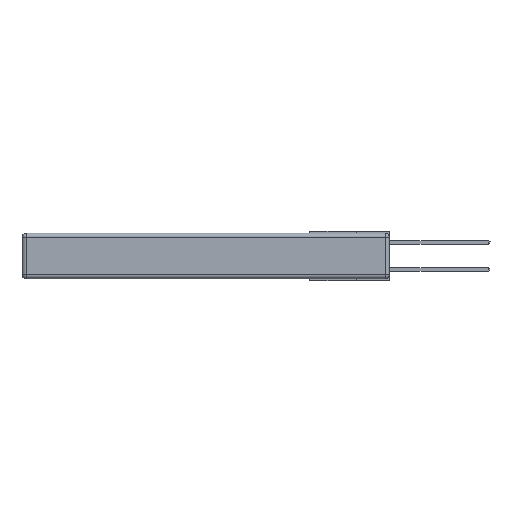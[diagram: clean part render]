
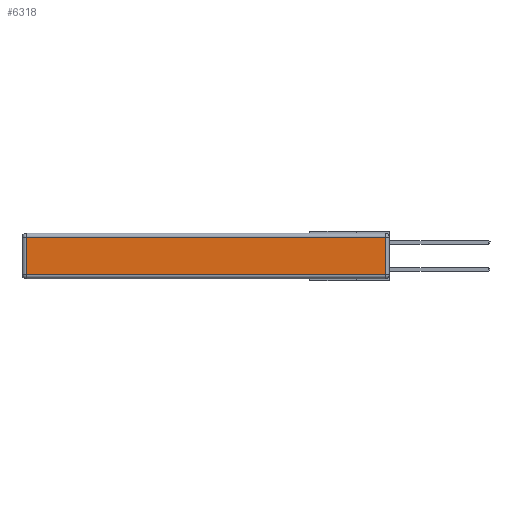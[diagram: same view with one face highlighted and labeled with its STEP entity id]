
A CAD part, left-side view. The second image highlights one B-rep face of the part: STEP entity #6318.
In plain terms, the highlighted planar face has unit normal (-1, 0, 0).
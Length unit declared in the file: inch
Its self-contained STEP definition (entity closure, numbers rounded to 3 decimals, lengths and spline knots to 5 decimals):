
#232 = DIRECTION ( 'NONE',  ( -1., 0., 0. ) ) ;
#442 = AXIS2_PLACEMENT_3D ( 'NONE', #15567, #232, #3858 ) ;
#449 = VECTOR ( 'NONE', #12687, 39.37008 ) ;
#954 = DIRECTION ( 'NONE',  ( 0., 0., -1. ) ) ;
#2299 = VERTEX_POINT ( 'NONE', #6662 ) ;
#2398 = CARTESIAN_POINT ( 'NONE',  ( 0., 0., -0.313 ) ) ;
#2404 = CARTESIAN_POINT ( 'NONE',  ( 0., 2.72, -0.343 ) ) ;
#2431 = EDGE_CURVE ( 'NONE', #2299, #5379, #15868, .T. ) ;
#3386 = FACE_OUTER_BOUND ( 'NONE', #5358, .T. ) ;
#3858 = DIRECTION ( 'NONE',  ( 0., 0., 1. ) ) ;
#4291 = DIRECTION ( 'NONE',  ( 0., 1., 0. ) ) ;
#4744 = EDGE_CURVE ( 'NONE', #13904, #5385, #16327, .T. ) ;
#4854 = EDGE_CURVE ( 'NONE', #5385, #2299, #6262, .T. ) ;
#5204 = PLANE ( 'NONE',  #442 ) ;
#5358 = EDGE_LOOP ( 'NONE', ( #5891, #11018, #9616, #16055 ) ) ;
#5379 = VERTEX_POINT ( 'NONE', #16578 ) ;
#5385 = VERTEX_POINT ( 'NONE', #16473 ) ;
#5401 = DIRECTION ( 'NONE',  ( 0., 0., 1. ) ) ;
#5891 = ORIENTED_EDGE ( 'NONE', *, *, #4744, .T. ) ;
#6262 = LINE ( 'NONE', #11719, #15922 ) ;
#6318 = ADVANCED_FACE ( 'NONE', ( #3386 ), #5204, .T. ) ;
#6662 = CARTESIAN_POINT ( 'NONE',  ( 0., 0.03, -0.03 ) ) ;
#8704 = LINE ( 'NONE', #2404, #9716 ) ;
#9384 = CARTESIAN_POINT ( 'NONE',  ( 0., 2.75, -0.03 ) ) ;
#9616 = ORIENTED_EDGE ( 'NONE', *, *, #2431, .T. ) ;
#9716 = VECTOR ( 'NONE', #954, 39.37008 ) ;
#11018 = ORIENTED_EDGE ( 'NONE', *, *, #4854, .T. ) ;
#11719 = CARTESIAN_POINT ( 'NONE',  ( 0., 0.03, -0.343 ) ) ;
#11794 = VECTOR ( 'NONE', #4291, 39.37008 ) ;
#12687 = DIRECTION ( 'NONE',  ( 0., -1., 0. ) ) ;
#13817 = CARTESIAN_POINT ( 'NONE',  ( 0., 2.72, -0.313 ) ) ;
#13904 = VERTEX_POINT ( 'NONE', #13817 ) ;
#15475 = EDGE_CURVE ( 'NONE', #5379, #13904, #8704, .T. ) ;
#15567 = CARTESIAN_POINT ( 'NONE',  ( 0., 0., -0.343 ) ) ;
#15868 = LINE ( 'NONE', #9384, #11794 ) ;
#15922 = VECTOR ( 'NONE', #5401, 39.37008 ) ;
#16055 = ORIENTED_EDGE ( 'NONE', *, *, #15475, .T. ) ;
#16327 = LINE ( 'NONE', #2398, #449 ) ;
#16473 = CARTESIAN_POINT ( 'NONE',  ( 0., 0.03, -0.313 ) ) ;
#16578 = CARTESIAN_POINT ( 'NONE',  ( 0., 2.72, -0.03 ) ) ;
